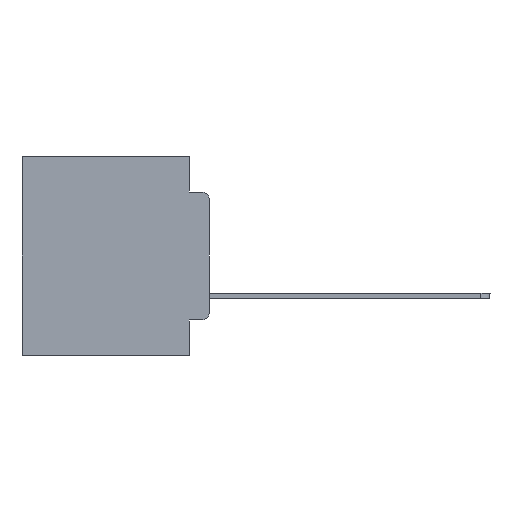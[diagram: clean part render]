
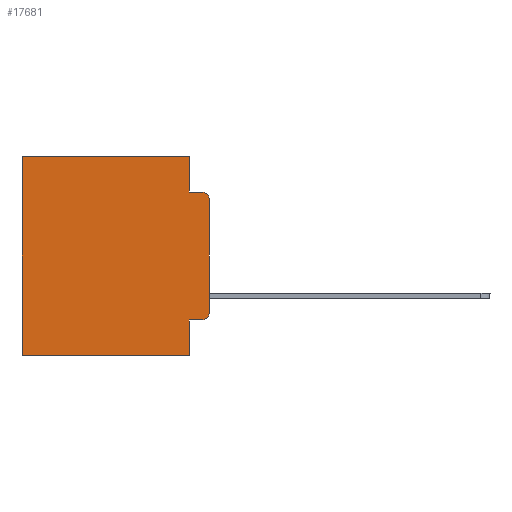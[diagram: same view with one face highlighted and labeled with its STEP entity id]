
A CAD part, left-side view. The second image highlights one B-rep face of the part: STEP entity #17681.
In plain terms, the highlighted planar face has unit normal (-1, 0, 0).
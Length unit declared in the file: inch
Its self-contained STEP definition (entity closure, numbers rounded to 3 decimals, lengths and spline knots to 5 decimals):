
#5 = CARTESIAN_POINT ( 'NONE',  ( 0.298, 0., -0.3915 ) ) ;
#82 = EDGE_CURVE ( 'NONE', #7473, #15913, #17184, .T. ) ;
#105 = ORIENTED_EDGE ( 'NONE', *, *, #82, .T. ) ;
#505 = DIRECTION ( 'NONE',  ( 0., 0., -1. ) ) ;
#1276 = FACE_OUTER_BOUND ( 'NONE', #6647, .T. ) ;
#1487 = DIRECTION ( 'NONE',  ( 0., 0., -1. ) ) ;
#1558 = CARTESIAN_POINT ( 'NONE',  ( 0.298, 0.051, -0.4115 ) ) ;
#1953 = ORIENTED_EDGE ( 'NONE', *, *, #12508, .T. ) ;
#1962 = EDGE_CURVE ( 'NONE', #10956, #14302, #2788, .T. ) ;
#2010 = CARTESIAN_POINT ( 'NONE',  ( 0.298, 0.02, -0.4115 ) ) ;
#2580 = EDGE_CURVE ( 'NONE', #5715, #16368, #12546, .T. ) ;
#2762 = EDGE_CURVE ( 'NONE', #17485, #5764, #11587, .T. ) ;
#2788 = LINE ( 'NONE', #14842, #5033 ) ;
#2836 = CARTESIAN_POINT ( 'NONE',  ( 0.298, 0.051, 0. ) ) ;
#3389 = VECTOR ( 'NONE', #22856, 39.37008 ) ;
#3996 = LINE ( 'NONE', #24097, #10707 ) ;
#4212 = ORIENTED_EDGE ( 'NONE', *, *, #2762, .F. ) ;
#4255 = ORIENTED_EDGE ( 'NONE', *, *, #16920, .F. ) ;
#4303 = CARTESIAN_POINT ( 'NONE',  ( 0.298, 0.02, -0.1085 ) ) ;
#4333 = CARTESIAN_POINT ( 'NONE',  ( 0.298, 0.051, -0.5 ) ) ;
#5033 = VECTOR ( 'NONE', #20661, 39.37008 ) ;
#5187 = CARTESIAN_POINT ( 'NONE',  ( 0.298, 0.02, -0.0885 ) ) ;
#5471 = CARTESIAN_POINT ( 'NONE',  ( 0.298, 0., 0. ) ) ;
#5715 = VERTEX_POINT ( 'NONE', #9190 ) ;
#5734 = DIRECTION ( 'NONE',  ( 0., 0., -1. ) ) ;
#5764 = VERTEX_POINT ( 'NONE', #18202 ) ;
#6267 = VERTEX_POINT ( 'NONE', #18023 ) ;
#6647 = EDGE_LOOP ( 'NONE', ( #4255, #1953, #7967, #25382, #15114, #10210, #4212, #20908, #20721, #105 ) ) ;
#7385 = EDGE_CURVE ( 'NONE', #16197, #7473, #3996, .T. ) ;
#7473 = VERTEX_POINT ( 'NONE', #2010 ) ;
#7700 = LINE ( 'NONE', #5471, #9895 ) ;
#7931 = VECTOR ( 'NONE', #25770, 39.37008 ) ;
#7967 = ORIENTED_EDGE ( 'NONE', *, *, #1962, .F. ) ;
#9076 = DIRECTION ( 'NONE',  ( 0., 0., -1. ) ) ;
#9190 = CARTESIAN_POINT ( 'NONE',  ( 0.298, 0.051, 0. ) ) ;
#9895 = VECTOR ( 'NONE', #1487, 39.37008 ) ;
#10210 = ORIENTED_EDGE ( 'NONE', *, *, #19465, .T. ) ;
#10707 = VECTOR ( 'NONE', #11929, 39.37008 ) ;
#10861 = DIRECTION ( 'NONE',  ( 0., 0., -1. ) ) ;
#10956 = VERTEX_POINT ( 'NONE', #21214 ) ;
#11587 = LINE ( 'NONE', #20075, #16068 ) ;
#11929 = DIRECTION ( 'NONE',  ( 0., -1., 0. ) ) ;
#12237 = DIRECTION ( 'NONE',  ( -1., 0., 0. ) ) ;
#12508 = EDGE_CURVE ( 'NONE', #6267, #14302, #15174, .T. ) ;
#12546 = LINE ( 'NONE', #20624, #3389 ) ;
#12772 = DIRECTION ( 'NONE',  ( 0., 0., -1. ) ) ;
#12994 = VECTOR ( 'NONE', #5734, 39.37008 ) ;
#13060 = CARTESIAN_POINT ( 'NONE',  ( 0.298, 0., 0. ) ) ;
#14302 = VERTEX_POINT ( 'NONE', #5187 ) ;
#14409 = CARTESIAN_POINT ( 'NONE',  ( 0.298, 0.473, 0. ) ) ;
#14842 = CARTESIAN_POINT ( 'NONE',  ( 0.298, 0.051, -0.0885 ) ) ;
#15114 = ORIENTED_EDGE ( 'NONE', *, *, #2580, .T. ) ;
#15174 = CIRCLE ( 'NONE', #16869, 0.02 ) ;
#15913 = VERTEX_POINT ( 'NONE', #5 ) ;
#15917 = CARTESIAN_POINT ( 'NONE',  ( 0.298, 0.473, 0. ) ) ;
#16068 = VECTOR ( 'NONE', #19683, 39.37008 ) ;
#16197 = VERTEX_POINT ( 'NONE', #1558 ) ;
#16368 = VERTEX_POINT ( 'NONE', #14409 ) ;
#16739 = LINE ( 'NONE', #2836, #22623 ) ;
#16869 = AXIS2_PLACEMENT_3D ( 'NONE', #4303, #12237, #10861 ) ;
#16920 = EDGE_CURVE ( 'NONE', #6267, #15913, #7700, .T. ) ;
#17136 = AXIS2_PLACEMENT_3D ( 'NONE', #13060, #22833, #9076 ) ;
#17184 = CIRCLE ( 'NONE', #24350, 0.02 ) ;
#17485 = VERTEX_POINT ( 'NONE', #4333 ) ;
#17681 = ADVANCED_FACE ( 'NONE', ( #1276 ), #20986, .F. ) ;
#17717 = LINE ( 'NONE', #23776, #7931 ) ;
#17799 = LINE ( 'NONE', #15917, #12994 ) ;
#17954 = EDGE_CURVE ( 'NONE', #16197, #17485, #16739, .T. ) ;
#18023 = CARTESIAN_POINT ( 'NONE',  ( 0.298, 0., -0.1085 ) ) ;
#18202 = CARTESIAN_POINT ( 'NONE',  ( 0.298, 0.473, -0.5 ) ) ;
#19465 = EDGE_CURVE ( 'NONE', #16368, #5764, #17799, .T. ) ;
#19683 = DIRECTION ( 'NONE',  ( 0., 1., 0. ) ) ;
#20075 = CARTESIAN_POINT ( 'NONE',  ( 0.298, 0., -0.5 ) ) ;
#20408 = EDGE_CURVE ( 'NONE', #5715, #10956, #17717, .T. ) ;
#20624 = CARTESIAN_POINT ( 'NONE',  ( 0.298, 0., 0. ) ) ;
#20661 = DIRECTION ( 'NONE',  ( 0., -1., 0. ) ) ;
#20721 = ORIENTED_EDGE ( 'NONE', *, *, #7385, .T. ) ;
#20753 = CARTESIAN_POINT ( 'NONE',  ( 0.298, 0.02, -0.3915 ) ) ;
#20908 = ORIENTED_EDGE ( 'NONE', *, *, #17954, .F. ) ;
#20986 = PLANE ( 'NONE',  #17136 ) ;
#21214 = CARTESIAN_POINT ( 'NONE',  ( 0.298, 0.051, -0.0885 ) ) ;
#22623 = VECTOR ( 'NONE', #12772, 39.37008 ) ;
#22833 = DIRECTION ( 'NONE',  ( 1., 0., 0. ) ) ;
#22856 = DIRECTION ( 'NONE',  ( 0., 1., 0. ) ) ;
#23776 = CARTESIAN_POINT ( 'NONE',  ( 0.298, 0.051, 0. ) ) ;
#24097 = CARTESIAN_POINT ( 'NONE',  ( 0.298, 0.051, -0.4115 ) ) ;
#24350 = AXIS2_PLACEMENT_3D ( 'NONE', #20753, #24701, #505 ) ;
#24701 = DIRECTION ( 'NONE',  ( -1., 0., 0. ) ) ;
#25382 = ORIENTED_EDGE ( 'NONE', *, *, #20408, .F. ) ;
#25770 = DIRECTION ( 'NONE',  ( 0., 0., -1. ) ) ;
